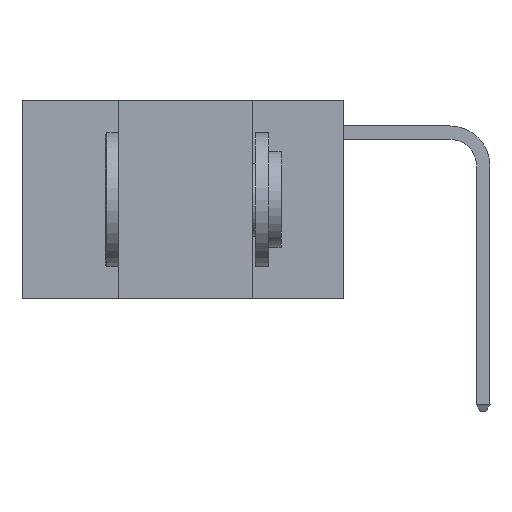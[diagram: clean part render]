
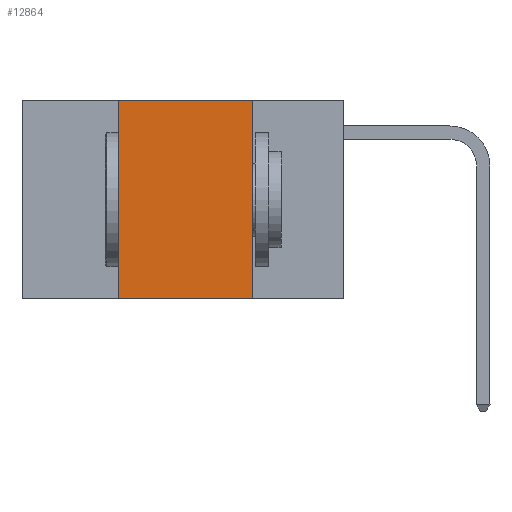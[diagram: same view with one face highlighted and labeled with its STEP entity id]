
A CAD part, left-side view. The second image highlights one B-rep face of the part: STEP entity #12864.
In plain terms, the highlighted planar face has unit normal (-1, 0, 0).
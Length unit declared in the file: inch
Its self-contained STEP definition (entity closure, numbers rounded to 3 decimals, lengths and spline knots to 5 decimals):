
#1376 = DIRECTION ( 'NONE',  ( 0., -1., 0. ) ) ;
#1714 = VECTOR ( 'NONE', #6286, 39.37008 ) ;
#2373 = VECTOR ( 'NONE', #2938, 39.37008 ) ;
#2938 = DIRECTION ( 'NONE',  ( 0., 0., 1. ) ) ;
#3307 = VECTOR ( 'NONE', #10114, 39.37008 ) ;
#3597 = ORIENTED_EDGE ( 'NONE', *, *, #11185, .F. ) ;
#4442 = ORIENTED_EDGE ( 'NONE', *, *, #13872, .F. ) ;
#4716 = FACE_OUTER_BOUND ( 'NONE', #18460, .T. ) ;
#5921 = LINE ( 'NONE', #10977, #1714 ) ;
#6024 = ORIENTED_EDGE ( 'NONE', *, *, #6896, .F. ) ;
#6126 = VERTEX_POINT ( 'NONE', #14740 ) ;
#6205 = ORIENTED_EDGE ( 'NONE', *, *, #13209, .T. ) ;
#6286 = DIRECTION ( 'NONE',  ( 0., -1., 0. ) ) ;
#6896 = EDGE_CURVE ( 'NONE', #8078, #7582, #14744, .T. ) ;
#7582 = VERTEX_POINT ( 'NONE', #19297 ) ;
#8078 = VERTEX_POINT ( 'NONE', #10092 ) ;
#8344 = DIRECTION ( 'NONE',  ( 0., 0., -1. ) ) ;
#9372 = VECTOR ( 'NONE', #1376, 39.37008 ) ;
#10092 = CARTESIAN_POINT ( 'NONE',  ( 0., 0.42, -0.37 ) ) ;
#10114 = DIRECTION ( 'NONE',  ( 0., 0., -1. ) ) ;
#10481 = AXIS2_PLACEMENT_3D ( 'NONE', #15938, #17486, #8344 ) ;
#10977 = CARTESIAN_POINT ( 'NONE',  ( 0., 0.6, 0. ) ) ;
#11185 = EDGE_CURVE ( 'NONE', #16397, #6126, #16129, .T. ) ;
#12277 = CARTESIAN_POINT ( 'NONE',  ( 0., 0.42, 0. ) ) ;
#12864 = ADVANCED_FACE ( 'NONE', ( #4716 ), #14414, .F. ) ;
#13209 = EDGE_CURVE ( 'NONE', #8078, #6126, #17953, .T. ) ;
#13872 = EDGE_CURVE ( 'NONE', #7582, #16397, #5921, .T. ) ;
#14414 = PLANE ( 'NONE',  #10481 ) ;
#14740 = CARTESIAN_POINT ( 'NONE',  ( 0., 0.17, -0.37 ) ) ;
#14744 = LINE ( 'NONE', #12277, #2373 ) ;
#15730 = CARTESIAN_POINT ( 'NONE',  ( 0., 0.17, 0. ) ) ;
#15938 = CARTESIAN_POINT ( 'NONE',  ( 0., 0.6, 0. ) ) ;
#16129 = LINE ( 'NONE', #17679, #3307 ) ;
#16397 = VERTEX_POINT ( 'NONE', #15730 ) ;
#17486 = DIRECTION ( 'NONE',  ( 1., 0., 0. ) ) ;
#17679 = CARTESIAN_POINT ( 'NONE',  ( 0., 0.17, 0. ) ) ;
#17953 = LINE ( 'NONE', #19906, #9372 ) ;
#18460 = EDGE_LOOP ( 'NONE', ( #3597, #4442, #6024, #6205 ) ) ;
#19297 = CARTESIAN_POINT ( 'NONE',  ( 0., 0.42, 0. ) ) ;
#19906 = CARTESIAN_POINT ( 'NONE',  ( 0., 0.6, -0.37 ) ) ;
